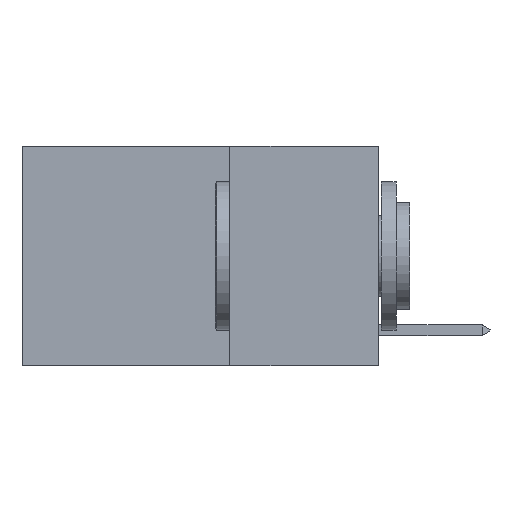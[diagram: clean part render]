
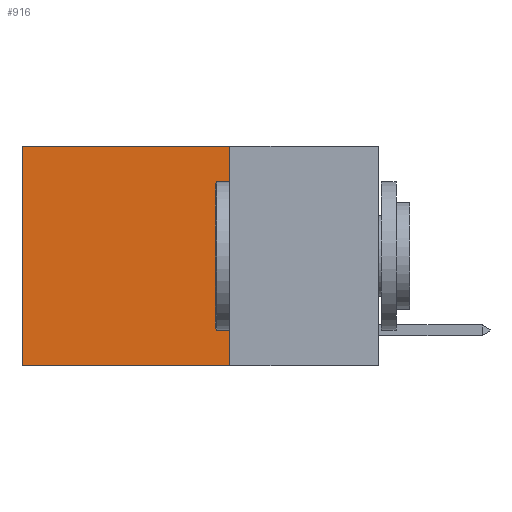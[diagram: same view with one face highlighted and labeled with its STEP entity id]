
A CAD part, left-side view. The second image highlights one B-rep face of the part: STEP entity #916.
In plain terms, the highlighted planar face has unit normal (-1, 0, 0).
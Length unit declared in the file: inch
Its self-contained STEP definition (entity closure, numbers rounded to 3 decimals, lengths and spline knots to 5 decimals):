
#143 = VECTOR ( 'NONE', #13247, 39.37008 ) ;
#318 = VERTEX_POINT ( 'NONE', #1935 ) ;
#650 = CARTESIAN_POINT ( 'NONE',  ( 0.2625, 0.25, 0. ) ) ;
#916 = ADVANCED_FACE ( 'NONE', ( #11217 ), #9958, .F. ) ;
#1135 = VERTEX_POINT ( 'NONE', #13944 ) ;
#1401 = LINE ( 'NONE', #8559, #14829 ) ;
#1935 = CARTESIAN_POINT ( 'NONE',  ( 0.2625, 0.6, -0.37 ) ) ;
#2031 = CARTESIAN_POINT ( 'NONE',  ( 0.2625, 0.25, 0. ) ) ;
#2343 = EDGE_CURVE ( 'NONE', #1135, #318, #5996, .T. ) ;
#2840 = ORIENTED_EDGE ( 'NONE', *, *, #4726, .T. ) ;
#3981 = DIRECTION ( 'NONE',  ( 0., 0., -1. ) ) ;
#4106 = AXIS2_PLACEMENT_3D ( 'NONE', #650, #14789, #3981 ) ;
#4726 = EDGE_CURVE ( 'NONE', #10388, #11736, #4905, .T. ) ;
#4905 = LINE ( 'NONE', #8440, #143 ) ;
#5996 = LINE ( 'NONE', #7263, #15235 ) ;
#6989 = EDGE_LOOP ( 'NONE', ( #10590, #8819, #12569, #2840 ) ) ;
#7028 = DIRECTION ( 'NONE',  ( 0., 1., 0. ) ) ;
#7263 = CARTESIAN_POINT ( 'NONE',  ( 0.2625, 0.25, -0.37 ) ) ;
#8143 = CARTESIAN_POINT ( 'NONE',  ( 0.2625, 0.6, 0. ) ) ;
#8440 = CARTESIAN_POINT ( 'NONE',  ( 0.2625, 0.25, 0. ) ) ;
#8559 = CARTESIAN_POINT ( 'NONE',  ( 0.2625, 0.25, 0. ) ) ;
#8576 = VECTOR ( 'NONE', #13189, 39.37008 ) ;
#8819 = ORIENTED_EDGE ( 'NONE', *, *, #2343, .F. ) ;
#9605 = EDGE_CURVE ( 'NONE', #10388, #1135, #1401, .T. ) ;
#9958 = PLANE ( 'NONE',  #4106 ) ;
#10388 = VERTEX_POINT ( 'NONE', #2031 ) ;
#10590 = ORIENTED_EDGE ( 'NONE', *, *, #12906, .T. ) ;
#11217 = FACE_OUTER_BOUND ( 'NONE', #6989, .T. ) ;
#11736 = VERTEX_POINT ( 'NONE', #15565 ) ;
#12569 = ORIENTED_EDGE ( 'NONE', *, *, #9605, .F. ) ;
#12906 = EDGE_CURVE ( 'NONE', #11736, #318, #13105, .T. ) ;
#13105 = LINE ( 'NONE', #8143, #8576 ) ;
#13189 = DIRECTION ( 'NONE',  ( 0., 0., -1. ) ) ;
#13247 = DIRECTION ( 'NONE',  ( 0., 1., 0. ) ) ;
#13301 = DIRECTION ( 'NONE',  ( 0., 0., -1. ) ) ;
#13944 = CARTESIAN_POINT ( 'NONE',  ( 0.2625, 0.25, -0.37 ) ) ;
#14789 = DIRECTION ( 'NONE',  ( 1., 0., 0. ) ) ;
#14829 = VECTOR ( 'NONE', #13301, 39.37008 ) ;
#15235 = VECTOR ( 'NONE', #7028, 39.37008 ) ;
#15565 = CARTESIAN_POINT ( 'NONE',  ( 0.2625, 0.6, 0. ) ) ;
